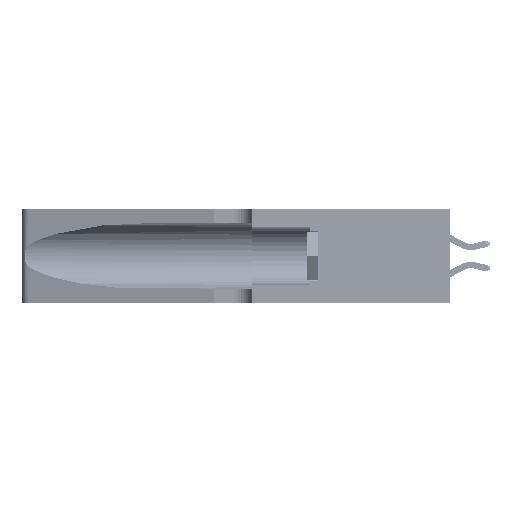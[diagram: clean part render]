
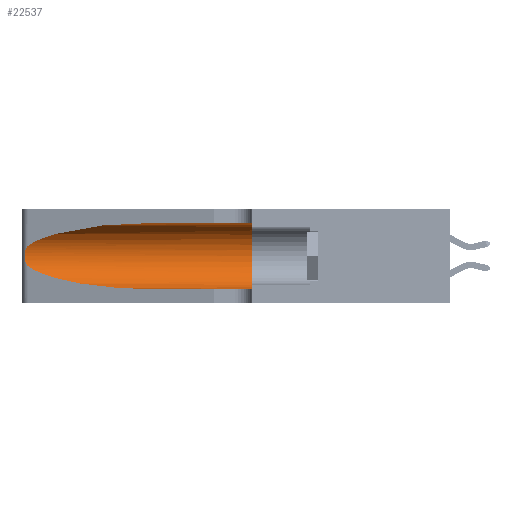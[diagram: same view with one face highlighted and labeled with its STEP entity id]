
A CAD part, left-side view. The second image highlights one B-rep face of the part: STEP entity #22537.
In plain terms, the highlighted cylindrical face has radius 3.308 mm (diameter 6.617 mm), a partial arc.
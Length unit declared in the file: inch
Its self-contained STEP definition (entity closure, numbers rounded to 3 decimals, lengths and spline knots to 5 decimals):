
#251 = VERTEX_POINT ( 'NONE', #43879 ) ;
#1196 = CARTESIAN_POINT ( 'NONE',  ( 0.18966, 0.96281, 0.05475 ) ) ;
#4008 = CARTESIAN_POINT ( 'NONE',  ( 0.25487, 1.22718, 0.14631 ) ) ;
#4691 = ORIENTED_EDGE ( 'NONE', *, *, #43230, .T. ) ;
#6412 = VERTEX_POINT ( 'NONE', #32068 ) ;
#6606 = ORIENTED_EDGE ( 'NONE', *, *, #21957, .F. ) ;
#7825 = CARTESIAN_POINT ( 'NONE',  ( 0.25789, 1.23486, 0.15765 ) ) ;
#8890 = LINE ( 'NONE', #24850, #19028 ) ;
#8916 = AXIS2_PLACEMENT_3D ( 'NONE', #20375, #9065, #12891 ) ;
#9065 = DIRECTION ( 'NONE',  ( 0., 1., 0. ) ) ;
#12891 = DIRECTION ( 'NONE',  ( 0., 0., 1. ) ) ;
#13086 = ORIENTED_EDGE ( 'NONE', *, *, #32517, .T. ) ;
#13106 = VERTEX_POINT ( 'NONE', #45585 ) ;
#13525 = DIRECTION ( 'NONE',  ( 0., -1., 0. ) ) ;
#14244 = EDGE_CURVE ( 'NONE', #13106, #251, #38799, .T. ) ;
#14484 =( BOUNDED_CURVE ( )  B_SPLINE_CURVE ( 3, ( #47844, #18297, #37165, #21613 ),
 .UNSPECIFIED., .F., .F. ) 
 B_SPLINE_CURVE_WITH_KNOTS ( ( 4, 4 ),
 ( 1.5708, 2.84003 ),
 .UNSPECIFIED. ) 
 CURVE ( )  GEOMETRIC_REPRESENTATION_ITEM ( )  RATIONAL_B_SPLINE_CURVE ( ( 1., 0.87, 0.87, 1. ) ) 
 REPRESENTATION_ITEM ( '' )  );
#14815 = CARTESIAN_POINT ( 'NONE',  ( 0.26017, 1.23833, 0.17102 ) ) ;
#15151 = CARTESIAN_POINT ( 'NONE',  ( 0.25555, 1.22993, 0.14849 ) ) ;
#18297 = CARTESIAN_POINT ( 'NONE',  ( 0.18966, 0.96281, 0.31525 ) ) ;
#18733 = ORIENTED_EDGE ( 'NONE', *, *, #14244, .T. ) ;
#18809 = CARTESIAN_POINT ( 'NONE',  ( 0.26075, 1.23896, 0.19203 ) ) ;
#18978 = CARTESIAN_POINT ( 'NONE',  ( 0.25854, 1.2359, 0.20912 ) ) ;
#19028 = VECTOR ( 'NONE', #44275, 39.37008 ) ;
#19906 = DIRECTION ( 'NONE',  ( 0., -1., 0. ) ) ;
#19967 = CARTESIAN_POINT ( 'NONE',  ( 0.25487, 1.22718, 0.14631 ) ) ;
#20375 = CARTESIAN_POINT ( 'NONE',  ( 0.1305, 0.35, 0.185 ) ) ;
#20453 = CARTESIAN_POINT ( 'NONE',  ( 0.2373, 1.15595, 0.08982 ) ) ;
#21613 = CARTESIAN_POINT ( 'NONE',  ( 0.25487, 1.22718, 0.22369 ) ) ;
#21957 = EDGE_CURVE ( 'NONE', #24760, #6412, #8890, .T. ) ;
#22453 = CARTESIAN_POINT ( 'NONE',  ( 0.26018, 1.23835, 0.19895 ) ) ;
#22537 = ADVANCED_FACE ( 'NONE', ( #30197 ), #33778, .F. ) ;
#24760 = VERTEX_POINT ( 'NONE', #25142 ) ;
#24850 = CARTESIAN_POINT ( 'NONE',  ( 0.1305, 1.61858, 0.31525 ) ) ;
#25142 = CARTESIAN_POINT ( 'NONE',  ( 0.1305, 0.72297, 0.31525 ) ) ;
#28080 = ORIENTED_EDGE ( 'NONE', *, *, #39014, .T. ) ;
#28514 = VERTEX_POINT ( 'NONE', #46089 ) ;
#28750 = CARTESIAN_POINT ( 'NONE',  ( 0.1305, 1.61858, 0.185 ) ) ;
#29274 = VECTOR ( 'NONE', #19906, 39.37008 ) ;
#30039 = CARTESIAN_POINT ( 'NONE',  ( 0.25787, 1.23484, 0.2124 ) ) ;
#30197 = FACE_OUTER_BOUND ( 'NONE', #30517, .T. ) ;
#30383 = CARTESIAN_POINT ( 'NONE',  ( 0.25555, 1.22994, 0.2215 ) ) ;
#30517 = EDGE_LOOP ( 'NONE', ( #4691, #28080, #18733, #13086, #32875, #6606 ) ) ;
#32068 = CARTESIAN_POINT ( 'NONE',  ( 0.1305, 0.35, 0.31525 ) ) ;
#32107 = B_SPLINE_CURVE_WITH_KNOTS ( 'NONE', 3,
 ( #41347, #30383, #45183, #30039, #18978, #22453, #18809, #48987, #14815, #37371, #7825, #33867, #15151, #4008 ),
 .UNSPECIFIED., .F., .F.,
 ( 4, 2, 2, 2, 2, 2, 4 ),
 ( 0., 0.00027, 0.00053, 0.00107, 0.0016, 0.00187, 0.00214 ),
 .UNSPECIFIED. ) ;
#32517 = EDGE_CURVE ( 'NONE', #251, #28514, #35805, .T. ) ;
#32875 = ORIENTED_EDGE ( 'NONE', *, *, #34216, .F. ) ;
#33253 = VERTEX_POINT ( 'NONE', #41022 ) ;
#33778 = CYLINDRICAL_SURFACE ( 'NONE', #42670, 0.13025 ) ;
#33867 = CARTESIAN_POINT ( 'NONE',  ( 0.25639, 1.23186, 0.15144 ) ) ;
#34216 = EDGE_CURVE ( 'NONE', #6412, #28514, #46414, .T. ) ;
#35805 = LINE ( 'NONE', #42598, #29274 ) ;
#37165 = CARTESIAN_POINT ( 'NONE',  ( 0.2373, 1.15595, 0.28018 ) ) ;
#37371 = CARTESIAN_POINT ( 'NONE',  ( 0.25856, 1.23593, 0.16098 ) ) ;
#38799 =( BOUNDED_CURVE ( )  B_SPLINE_CURVE ( 3, ( #19967, #20453, #1196, #46825 ),
 .UNSPECIFIED., .F., .F. ) 
 B_SPLINE_CURVE_WITH_KNOTS ( ( 4, 4 ),
 ( 3.44316, 4.71239 ),
 .UNSPECIFIED. ) 
 CURVE ( )  GEOMETRIC_REPRESENTATION_ITEM ( )  RATIONAL_B_SPLINE_CURVE ( ( 1., 0.87, 0.87, 1. ) ) 
 REPRESENTATION_ITEM ( '' )  );
#39014 = EDGE_CURVE ( 'NONE', #33253, #13106, #32107, .T. ) ;
#41022 = CARTESIAN_POINT ( 'NONE',  ( 0.25487, 1.22718, 0.22369 ) ) ;
#41347 = CARTESIAN_POINT ( 'NONE',  ( 0.25487, 1.22718, 0.22369 ) ) ;
#42598 = CARTESIAN_POINT ( 'NONE',  ( 0.1305, 1.61858, 0.05475 ) ) ;
#42670 = AXIS2_PLACEMENT_3D ( 'NONE', #28750, #13525, #43881 ) ;
#43230 = EDGE_CURVE ( 'NONE', #24760, #33253, #14484, .T. ) ;
#43879 = CARTESIAN_POINT ( 'NONE',  ( 0.1305, 0.72297, 0.05475 ) ) ;
#43881 = DIRECTION ( 'NONE',  ( 0., 0., -1. ) ) ;
#44275 = DIRECTION ( 'NONE',  ( 0., -1., 0. ) ) ;
#45183 = CARTESIAN_POINT ( 'NONE',  ( 0.25639, 1.23184, 0.21858 ) ) ;
#45585 = CARTESIAN_POINT ( 'NONE',  ( 0.25487, 1.22718, 0.14631 ) ) ;
#46089 = CARTESIAN_POINT ( 'NONE',  ( 0.1305, 0.35, 0.05475 ) ) ;
#46414 = CIRCLE ( 'NONE', #8916, 0.13025 ) ;
#46825 = CARTESIAN_POINT ( 'NONE',  ( 0.1305, 0.72297, 0.05475 ) ) ;
#47844 = CARTESIAN_POINT ( 'NONE',  ( 0.1305, 0.72297, 0.31525 ) ) ;
#48987 = CARTESIAN_POINT ( 'NONE',  ( 0.26075, 1.23896, 0.178 ) ) ;
